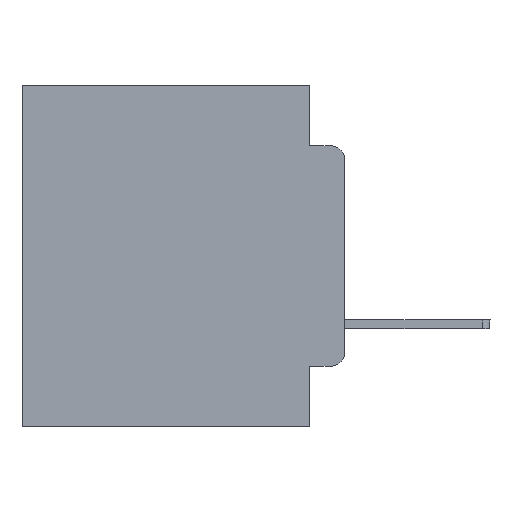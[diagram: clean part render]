
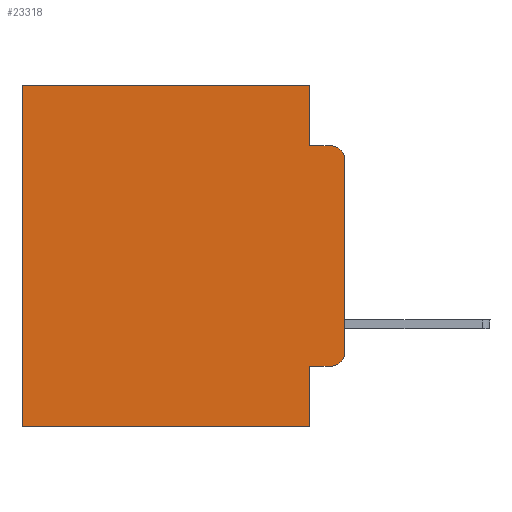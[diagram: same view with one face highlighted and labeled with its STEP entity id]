
A CAD part, left-side view. The second image highlights one B-rep face of the part: STEP entity #23318.
In plain terms, the highlighted planar face has unit normal (-1, 0, 0).
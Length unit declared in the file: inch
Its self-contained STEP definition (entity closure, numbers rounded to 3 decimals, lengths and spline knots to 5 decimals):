
#170 = VECTOR ( 'NONE', #23737, 39.37008 ) ;
#1176 = DIRECTION ( 'NONE',  ( -1., 0., 0. ) ) ;
#1618 = ORIENTED_EDGE ( 'NONE', *, *, #15385, .T. ) ;
#1656 = CARTESIAN_POINT ( 'NONE',  ( 0.298, 0.051, -0.0885 ) ) ;
#1928 = AXIS2_PLACEMENT_3D ( 'NONE', #19885, #19623, #17649 ) ;
#2398 = VERTEX_POINT ( 'NONE', #19064 ) ;
#2409 = ORIENTED_EDGE ( 'NONE', *, *, #9287, .F. ) ;
#2528 = VECTOR ( 'NONE', #11279, 39.37008 ) ;
#2761 = CIRCLE ( 'NONE', #4017, 0.02 ) ;
#2826 = ORIENTED_EDGE ( 'NONE', *, *, #8438, .F. ) ;
#3299 = EDGE_LOOP ( 'NONE', ( #2826, #1618, #13137, #10136, #26023, #19938, #18584, #2409, #3387, #23747 ) ) ;
#3387 = ORIENTED_EDGE ( 'NONE', *, *, #6717, .T. ) ;
#3424 = CARTESIAN_POINT ( 'NONE',  ( 0.298, 0., 0. ) ) ;
#4017 = AXIS2_PLACEMENT_3D ( 'NONE', #17582, #1176, #9632 ) ;
#4075 = CARTESIAN_POINT ( 'NONE',  ( 0.298, 0.02, -0.4115 ) ) ;
#4232 = CARTESIAN_POINT ( 'NONE',  ( 0.298, 0., -0.5 ) ) ;
#4831 = DIRECTION ( 'NONE',  ( 0., 0., -1. ) ) ;
#5056 = LINE ( 'NONE', #21080, #2528 ) ;
#5197 = CARTESIAN_POINT ( 'NONE',  ( 0.298, 0., 0. ) ) ;
#5376 = VERTEX_POINT ( 'NONE', #6643 ) ;
#5782 = EDGE_CURVE ( 'NONE', #23365, #5376, #22362, .T. ) ;
#6265 = CARTESIAN_POINT ( 'NONE',  ( 0.298, 0.02, -0.0885 ) ) ;
#6462 = CARTESIAN_POINT ( 'NONE',  ( 0.298, 0.473, 0. ) ) ;
#6545 = VERTEX_POINT ( 'NONE', #6265 ) ;
#6643 = CARTESIAN_POINT ( 'NONE',  ( 0.298, 0.473, -0.5 ) ) ;
#6717 = EDGE_CURVE ( 'NONE', #23299, #16855, #5056, .T. ) ;
#7190 = LINE ( 'NONE', #5197, #23865 ) ;
#7362 = DIRECTION ( 'NONE',  ( 0., 0., -1. ) ) ;
#7394 = DIRECTION ( 'NONE',  ( 0., 0., -1. ) ) ;
#7919 = LINE ( 'NONE', #3424, #9253 ) ;
#7991 = LINE ( 'NONE', #1656, #170 ) ;
#8190 = DIRECTION ( 'NONE',  ( 1., 0., 0. ) ) ;
#8333 = PLANE ( 'NONE',  #11111 ) ;
#8438 = EDGE_CURVE ( 'NONE', #25650, #11419, #7919, .T. ) ;
#9253 = VECTOR ( 'NONE', #17601, 39.37008 ) ;
#9287 = EDGE_CURVE ( 'NONE', #23299, #23365, #19420, .T. ) ;
#9344 = CARTESIAN_POINT ( 'NONE',  ( 0.298, 0.051, 0. ) ) ;
#9632 = DIRECTION ( 'NONE',  ( 0., 0., -1. ) ) ;
#9699 = VECTOR ( 'NONE', #7362, 39.37008 ) ;
#10136 = ORIENTED_EDGE ( 'NONE', *, *, #12115, .F. ) ;
#10167 = EDGE_CURVE ( 'NONE', #22106, #5376, #25531, .T. ) ;
#10694 = CARTESIAN_POINT ( 'NONE',  ( 0.298, 0., -0.1085 ) ) ;
#11111 = AXIS2_PLACEMENT_3D ( 'NONE', #17867, #8190, #22358 ) ;
#11279 = DIRECTION ( 'NONE',  ( 0., -1., 0. ) ) ;
#11419 = VERTEX_POINT ( 'NONE', #24069 ) ;
#12115 = EDGE_CURVE ( 'NONE', #17973, #2398, #20854, .T. ) ;
#12129 = CARTESIAN_POINT ( 'NONE',  ( 0.298, 0.051, 0. ) ) ;
#12301 = DIRECTION ( 'NONE',  ( 0., 1., 0. ) ) ;
#13137 = ORIENTED_EDGE ( 'NONE', *, *, #22824, .F. ) ;
#14568 = EDGE_CURVE ( 'NONE', #16855, #11419, #18819, .T. ) ;
#15385 = EDGE_CURVE ( 'NONE', #25650, #6545, #2761, .T. ) ;
#15613 = CARTESIAN_POINT ( 'NONE',  ( 0.298, 0.473, 0. ) ) ;
#15756 = EDGE_CURVE ( 'NONE', #17973, #22106, #7190, .T. ) ;
#16167 = VECTOR ( 'NONE', #12301, 39.37008 ) ;
#16855 = VERTEX_POINT ( 'NONE', #4075 ) ;
#16936 = CARTESIAN_POINT ( 'NONE',  ( 0.298, 0.051, -0.5 ) ) ;
#17582 = CARTESIAN_POINT ( 'NONE',  ( 0.298, 0.02, -0.1085 ) ) ;
#17601 = DIRECTION ( 'NONE',  ( 0., 0., -1. ) ) ;
#17649 = DIRECTION ( 'NONE',  ( 0., 0., -1. ) ) ;
#17867 = CARTESIAN_POINT ( 'NONE',  ( 0.298, 0., 0. ) ) ;
#17973 = VERTEX_POINT ( 'NONE', #12129 ) ;
#18584 = ORIENTED_EDGE ( 'NONE', *, *, #5782, .F. ) ;
#18819 = CIRCLE ( 'NONE', #1928, 0.02 ) ;
#19064 = CARTESIAN_POINT ( 'NONE',  ( 0.298, 0.051, -0.0885 ) ) ;
#19420 = LINE ( 'NONE', #9344, #9699 ) ;
#19623 = DIRECTION ( 'NONE',  ( -1., 0., 0. ) ) ;
#19885 = CARTESIAN_POINT ( 'NONE',  ( 0.298, 0.02, -0.3915 ) ) ;
#19938 = ORIENTED_EDGE ( 'NONE', *, *, #10167, .T. ) ;
#20125 = CARTESIAN_POINT ( 'NONE',  ( 0.298, 0.051, -0.4115 ) ) ;
#20383 = FACE_OUTER_BOUND ( 'NONE', #3299, .T. ) ;
#20854 = LINE ( 'NONE', #23109, #23037 ) ;
#21080 = CARTESIAN_POINT ( 'NONE',  ( 0.298, 0.051, -0.4115 ) ) ;
#21342 = DIRECTION ( 'NONE',  ( 0., 1., 0. ) ) ;
#22106 = VERTEX_POINT ( 'NONE', #6462 ) ;
#22358 = DIRECTION ( 'NONE',  ( 0., 0., -1. ) ) ;
#22362 = LINE ( 'NONE', #4232, #16167 ) ;
#22824 = EDGE_CURVE ( 'NONE', #2398, #6545, #7991, .T. ) ;
#23037 = VECTOR ( 'NONE', #4831, 39.37008 ) ;
#23109 = CARTESIAN_POINT ( 'NONE',  ( 0.298, 0.051, 0. ) ) ;
#23299 = VERTEX_POINT ( 'NONE', #20125 ) ;
#23318 = ADVANCED_FACE ( 'NONE', ( #20383 ), #8333, .F. ) ;
#23365 = VERTEX_POINT ( 'NONE', #16936 ) ;
#23737 = DIRECTION ( 'NONE',  ( 0., -1., 0. ) ) ;
#23747 = ORIENTED_EDGE ( 'NONE', *, *, #14568, .T. ) ;
#23865 = VECTOR ( 'NONE', #21342, 39.37008 ) ;
#24069 = CARTESIAN_POINT ( 'NONE',  ( 0.298, 0., -0.3915 ) ) ;
#25531 = LINE ( 'NONE', #15613, #25977 ) ;
#25650 = VERTEX_POINT ( 'NONE', #10694 ) ;
#25977 = VECTOR ( 'NONE', #7394, 39.37008 ) ;
#26023 = ORIENTED_EDGE ( 'NONE', *, *, #15756, .T. ) ;
